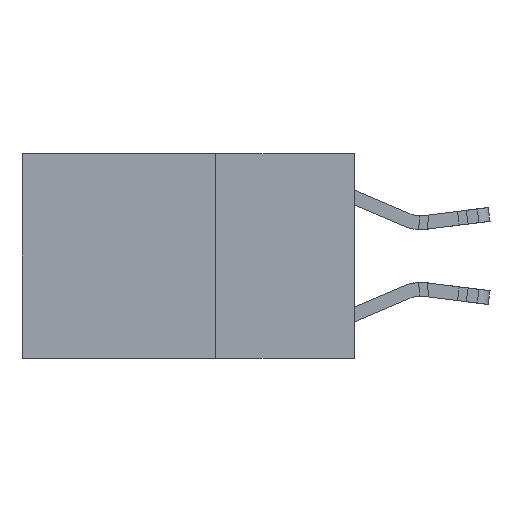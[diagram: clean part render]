
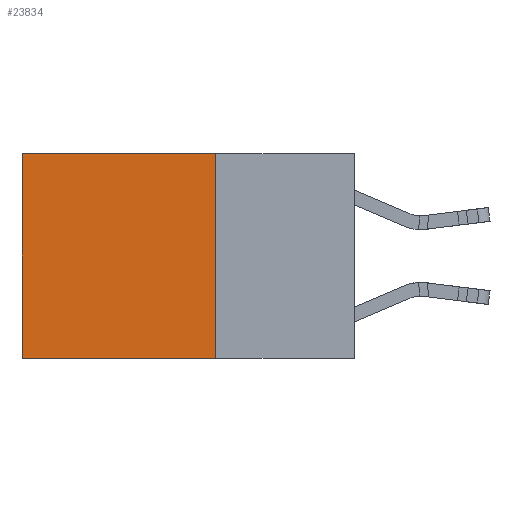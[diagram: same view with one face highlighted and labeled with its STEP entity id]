
A CAD part, left-side view. The second image highlights one B-rep face of the part: STEP entity #23834.
In plain terms, the highlighted planar face has unit normal (-1, 0, 0).
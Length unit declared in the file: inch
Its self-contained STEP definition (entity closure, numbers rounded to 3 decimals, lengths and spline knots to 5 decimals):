
#419 = EDGE_CURVE ( 'NONE', #23385, #3366, #3443, .T. ) ;
#1208 = EDGE_CURVE ( 'NONE', #3366, #1356, #21458, .T. ) ;
#1356 = VERTEX_POINT ( 'NONE', #19639 ) ;
#2230 = EDGE_CURVE ( 'NONE', #23385, #7562, #19678, .T. ) ;
#3366 = VERTEX_POINT ( 'NONE', #14177 ) ;
#3440 = ORIENTED_EDGE ( 'NONE', *, *, #2230, .F. ) ;
#3443 = LINE ( 'NONE', #12644, #11822 ) ;
#4708 = VECTOR ( 'NONE', #26926, 39.37008 ) ;
#4761 = DIRECTION ( 'NONE',  ( 0., 0., -1. ) ) ;
#5523 = EDGE_CURVE ( 'NONE', #7562, #1356, #7375, .T. ) ;
#7375 = LINE ( 'NONE', #16567, #11930 ) ;
#7562 = VERTEX_POINT ( 'NONE', #26920 ) ;
#10664 = CARTESIAN_POINT ( 'NONE',  ( 0.2625, 0.25, 0. ) ) ;
#11109 = DIRECTION ( 'NONE',  ( 1., 0., 0. ) ) ;
#11765 = AXIS2_PLACEMENT_3D ( 'NONE', #27086, #11109, #24674 ) ;
#11822 = VECTOR ( 'NONE', #21819, 39.37008 ) ;
#11930 = VECTOR ( 'NONE', #25773, 39.37008 ) ;
#12644 = CARTESIAN_POINT ( 'NONE',  ( 0.2625, 0.25, 0. ) ) ;
#13002 = CARTESIAN_POINT ( 'NONE',  ( 0.2625, 0.25, 0. ) ) ;
#14177 = CARTESIAN_POINT ( 'NONE',  ( 0.2625, 0.6, 0. ) ) ;
#16567 = CARTESIAN_POINT ( 'NONE',  ( 0.2625, 0.25, -0.37 ) ) ;
#18319 = PLANE ( 'NONE',  #11765 ) ;
#19639 = CARTESIAN_POINT ( 'NONE',  ( 0.2625, 0.6, -0.37 ) ) ;
#19678 = LINE ( 'NONE', #10664, #4708 ) ;
#21370 = ORIENTED_EDGE ( 'NONE', *, *, #419, .T. ) ;
#21458 = LINE ( 'NONE', #26007, #23425 ) ;
#21819 = DIRECTION ( 'NONE',  ( 0., 1., 0. ) ) ;
#23385 = VERTEX_POINT ( 'NONE', #13002 ) ;
#23425 = VECTOR ( 'NONE', #4761, 39.37008 ) ;
#23834 = ADVANCED_FACE ( 'NONE', ( #27226 ), #18319, .F. ) ;
#24674 = DIRECTION ( 'NONE',  ( 0., 0., -1. ) ) ;
#25000 = EDGE_LOOP ( 'NONE', ( #28704, #27024, #3440, #21370 ) ) ;
#25773 = DIRECTION ( 'NONE',  ( 0., 1., 0. ) ) ;
#26007 = CARTESIAN_POINT ( 'NONE',  ( 0.2625, 0.6, 0. ) ) ;
#26920 = CARTESIAN_POINT ( 'NONE',  ( 0.2625, 0.25, -0.37 ) ) ;
#26926 = DIRECTION ( 'NONE',  ( 0., 0., -1. ) ) ;
#27024 = ORIENTED_EDGE ( 'NONE', *, *, #5523, .F. ) ;
#27086 = CARTESIAN_POINT ( 'NONE',  ( 0.2625, 0.25, 0. ) ) ;
#27226 = FACE_OUTER_BOUND ( 'NONE', #25000, .T. ) ;
#28704 = ORIENTED_EDGE ( 'NONE', *, *, #1208, .T. ) ;
